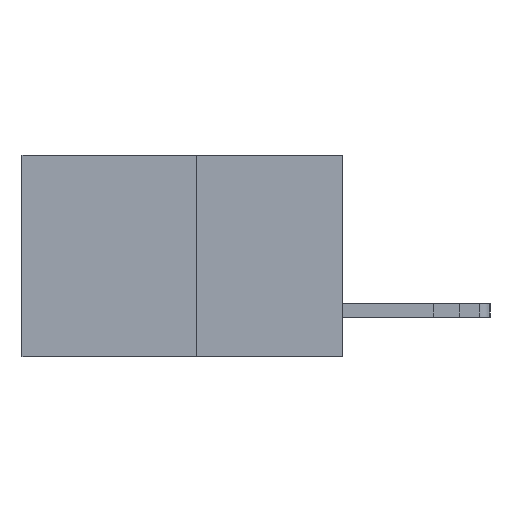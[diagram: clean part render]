
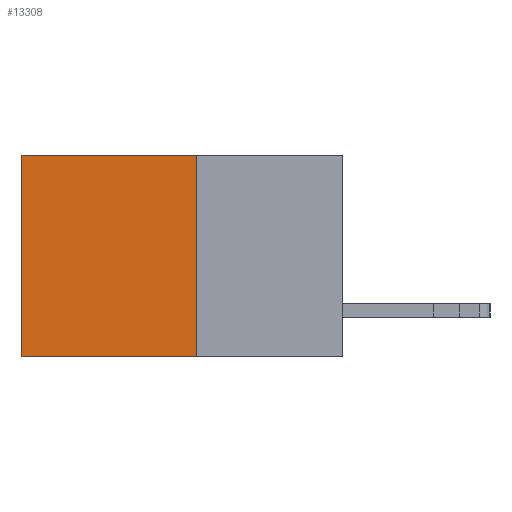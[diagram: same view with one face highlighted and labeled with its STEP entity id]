
A CAD part, left-side view. The second image highlights one B-rep face of the part: STEP entity #13308.
In plain terms, the highlighted planar face has unit normal (-1, 0, 0).
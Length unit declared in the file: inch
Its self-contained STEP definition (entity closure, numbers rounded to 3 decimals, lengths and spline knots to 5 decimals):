
#340 = VECTOR ( 'NONE', #11120, 39.37008 ) ;
#942 = CARTESIAN_POINT ( 'NONE',  ( 0.277, 0.27, -0.37 ) ) ;
#1385 = EDGE_LOOP ( 'NONE', ( #8827, #10543, #4537, #5773 ) ) ;
#1939 = EDGE_CURVE ( 'NONE', #2206, #10936, #2153, .T. ) ;
#2153 = LINE ( 'NONE', #10973, #10388 ) ;
#2206 = VERTEX_POINT ( 'NONE', #13279 ) ;
#2583 = DIRECTION ( 'NONE',  ( 1., 0., 0. ) ) ;
#2817 = AXIS2_PLACEMENT_3D ( 'NONE', #942, #2583, #14117 ) ;
#2902 = CARTESIAN_POINT ( 'NONE',  ( 0.277, 0.59, 0. ) ) ;
#3819 = EDGE_CURVE ( 'NONE', #10936, #10380, #20201, .T. ) ;
#4189 = LINE ( 'NONE', #7917, #340 ) ;
#4537 = ORIENTED_EDGE ( 'NONE', *, *, #16154, .F. ) ;
#5764 = LINE ( 'NONE', #5918, #10198 ) ;
#5773 = ORIENTED_EDGE ( 'NONE', *, *, #1939, .T. ) ;
#5918 = CARTESIAN_POINT ( 'NONE',  ( 0.277, 0.27, -0.37 ) ) ;
#7675 = DIRECTION ( 'NONE',  ( 0., 1., 0. ) ) ;
#7756 = VECTOR ( 'NONE', #17837, 39.37008 ) ;
#7879 = VERTEX_POINT ( 'NONE', #15134 ) ;
#7917 = CARTESIAN_POINT ( 'NONE',  ( 0.277, 0.27, -0.37 ) ) ;
#8827 = ORIENTED_EDGE ( 'NONE', *, *, #3819, .T. ) ;
#10198 = VECTOR ( 'NONE', #19092, 39.37008 ) ;
#10380 = VERTEX_POINT ( 'NONE', #20821 ) ;
#10388 = VECTOR ( 'NONE', #7675, 39.37008 ) ;
#10543 = ORIENTED_EDGE ( 'NONE', *, *, #19942, .F. ) ;
#10785 = PLANE ( 'NONE',  #2817 ) ;
#10936 = VERTEX_POINT ( 'NONE', #2902 ) ;
#10973 = CARTESIAN_POINT ( 'NONE',  ( 0.277, 0.27, 0. ) ) ;
#11120 = DIRECTION ( 'NONE',  ( 0., 0., -1. ) ) ;
#13279 = CARTESIAN_POINT ( 'NONE',  ( 0.277, 0.27, 0. ) ) ;
#13308 = ADVANCED_FACE ( 'NONE', ( #18436 ), #10785, .F. ) ;
#13467 = CARTESIAN_POINT ( 'NONE',  ( 0.277, 0.59, -0.37 ) ) ;
#14117 = DIRECTION ( 'NONE',  ( 0., 0., -1. ) ) ;
#15134 = CARTESIAN_POINT ( 'NONE',  ( 0.277, 0.27, -0.37 ) ) ;
#16154 = EDGE_CURVE ( 'NONE', #2206, #7879, #4189, .T. ) ;
#17837 = DIRECTION ( 'NONE',  ( 0., 0., -1. ) ) ;
#18436 = FACE_OUTER_BOUND ( 'NONE', #1385, .T. ) ;
#19092 = DIRECTION ( 'NONE',  ( 0., 1., 0. ) ) ;
#19942 = EDGE_CURVE ( 'NONE', #7879, #10380, #5764, .T. ) ;
#20201 = LINE ( 'NONE', #13467, #7756 ) ;
#20821 = CARTESIAN_POINT ( 'NONE',  ( 0.277, 0.59, -0.37 ) ) ;
